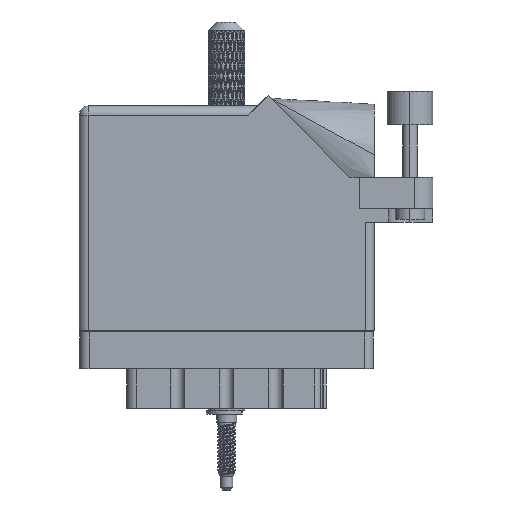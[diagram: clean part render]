
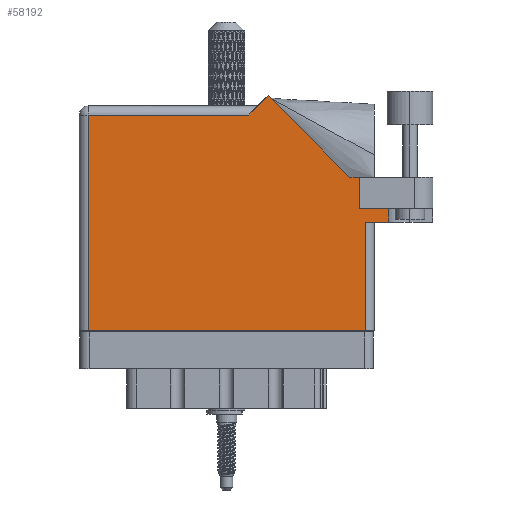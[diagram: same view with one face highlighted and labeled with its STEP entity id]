
A CAD part, front view. The second image highlights one B-rep face of the part: STEP entity #58192.
In plain terms, the highlighted face is planar.
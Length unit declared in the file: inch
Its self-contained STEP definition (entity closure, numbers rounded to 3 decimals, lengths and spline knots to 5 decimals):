
#96 = VECTOR ( 'NONE', #58342, 39.37008 ) ;
#247 = EDGE_CURVE ( 'NONE', #43957, #99186, #44743, .T. ) ;
#1475 = VERTEX_POINT ( 'NONE', #89538 ) ;
#3859 = LINE ( 'NONE', #57505, #86790 ) ;
#4360 = VECTOR ( 'NONE', #66414, 39.37008 ) ;
#4666 = CARTESIAN_POINT ( 'NONE',  ( 1.948, 0.737, 0. ) ) ;
#5744 = VERTEX_POINT ( 'NONE', #47094 ) ;
#8907 = CARTESIAN_POINT ( 'NONE',  ( 0.062, 0., 0. ) ) ;
#10261 = CARTESIAN_POINT ( 'NONE',  ( 2.41, 1.044, 0. ) ) ;
#13015 = DIRECTION ( 'NONE',  ( 0., 1., 0. ) ) ;
#15179 = CARTESIAN_POINT ( 'NONE',  ( 1.948, 0.737, 0. ) ) ;
#17141 = CARTESIAN_POINT ( 'NONE',  ( 1.155, 1.468, 0. ) ) ;
#17288 = VECTOR ( 'NONE', #83470, 39.37008 ) ;
#17927 = ORIENTED_EDGE ( 'NONE', *, *, #98427, .F. ) ;
#19640 = LINE ( 'NONE', #77623, #62447 ) ;
#21634 = ORIENTED_EDGE ( 'NONE', *, *, #247, .T. ) ;
#21904 = CARTESIAN_POINT ( 'NONE',  ( 0., 0., 0. ) ) ;
#21919 = VECTOR ( 'NONE', #69348, 39.37008 ) ;
#23807 = CARTESIAN_POINT ( 'NONE',  ( 1.28771, 1.60071, 0. ) ) ;
#26473 = CARTESIAN_POINT ( 'NONE',  ( 1.91, 0.831, 0. ) ) ;
#26623 = AXIS2_PLACEMENT_3D ( 'NONE', #48962, #105425, #56221 ) ;
#26885 = EDGE_CURVE ( 'NONE', #1475, #105498, #107430, .T. ) ;
#27562 = DIRECTION ( 'NONE',  ( -0.707, -0.707, 0. ) ) ;
#28063 = LINE ( 'NONE', #89338, #53928 ) ;
#28598 = ORIENTED_EDGE ( 'NONE', *, *, #95129, .T. ) ;
#28886 = CARTESIAN_POINT ( 'NONE',  ( 1.84442, 1.044, 0. ) ) ;
#30635 = LINE ( 'NONE', #65746, #93976 ) ;
#32898 = ORIENTED_EDGE ( 'NONE', *, *, #69110, .F. ) ;
#33162 = DIRECTION ( 'NONE',  ( 0., -1., 0. ) ) ;
#34593 = VERTEX_POINT ( 'NONE', #17141 ) ;
#36619 = CARTESIAN_POINT ( 'NONE',  ( 1.217, 1.53, 0. ) ) ;
#37528 = DIRECTION ( 'NONE',  ( 1., 0., 0. ) ) ;
#42921 = VECTOR ( 'NONE', #37528, 39.37008 ) ;
#43957 = VERTEX_POINT ( 'NONE', #69590 ) ;
#44743 = LINE ( 'NONE', #4666, #57774 ) ;
#45487 = LINE ( 'NONE', #21904, #42921 ) ;
#45895 = EDGE_CURVE ( 'NONE', #105498, #94994, #79507, .T. ) ;
#47094 = CARTESIAN_POINT ( 'NONE',  ( 0.062, 1.468, 0. ) ) ;
#47248 = FACE_OUTER_BOUND ( 'NONE', #101549, .T. ) ;
#48962 = CARTESIAN_POINT ( 'NONE',  ( 0., 1.53, 0. ) ) ;
#50933 = ORIENTED_EDGE ( 'NONE', *, *, #80934, .T. ) ;
#52217 = VERTEX_POINT ( 'NONE', #100976 ) ;
#53928 = VECTOR ( 'NONE', #88274, 39.37008 ) ;
#54864 = LINE ( 'NONE', #88343, #96 ) ;
#55256 = EDGE_CURVE ( 'NONE', #94994, #34593, #92895, .T. ) ;
#55393 = VERTEX_POINT ( 'NONE', #55421 ) ;
#55421 = CARTESIAN_POINT ( 'NONE',  ( 2.1115, 0.737, 0. ) ) ;
#56221 = DIRECTION ( 'NONE',  ( -1., 0., 0. ) ) ;
#57505 = CARTESIAN_POINT ( 'NONE',  ( 1.91, 0.831, 0. ) ) ;
#57774 = VECTOR ( 'NONE', #13015, 39.37008 ) ;
#58192 = ADVANCED_FACE ( 'NONE', ( #47248 ), #71475, .F. ) ;
#58342 = DIRECTION ( 'NONE',  ( 0., 1., 0. ) ) ;
#58554 = ORIENTED_EDGE ( 'NONE', *, *, #105888, .T. ) ;
#62447 = VECTOR ( 'NONE', #70772, 39.37008 ) ;
#65503 = ORIENTED_EDGE ( 'NONE', *, *, #86765, .T. ) ;
#65746 = CARTESIAN_POINT ( 'NONE',  ( 0.062, 0., 0. ) ) ;
#66414 = DIRECTION ( 'NONE',  ( -0.707, 0.707, 0. ) ) ;
#69110 = EDGE_CURVE ( 'NONE', #52217, #55393, #28063, .T. ) ;
#69348 = DIRECTION ( 'NONE',  ( -1., 0., 0. ) ) ;
#69590 = CARTESIAN_POINT ( 'NONE',  ( 1.948, 0., 0. ) ) ;
#70772 = DIRECTION ( 'NONE',  ( -1., 0., 0. ) ) ;
#70841 = ORIENTED_EDGE ( 'NONE', *, *, #26885, .T. ) ;
#71445 = VERTEX_POINT ( 'NONE', #8907 ) ;
#71475 = PLANE ( 'NONE',  #26623 ) ;
#77623 = CARTESIAN_POINT ( 'NONE',  ( 0., 1.468, 0. ) ) ;
#79507 = LINE ( 'NONE', #100362, #4360 ) ;
#80934 = EDGE_CURVE ( 'NONE', #71445, #43957, #45487, .T. ) ;
#82495 = VECTOR ( 'NONE', #27562, 39.37008 ) ;
#83470 = DIRECTION ( 'NONE',  ( 1., 0., 0. ) ) ;
#86765 = EDGE_CURVE ( 'NONE', #5744, #71445, #30635, .T. ) ;
#86790 = VECTOR ( 'NONE', #90725, 39.37008 ) ;
#88274 = DIRECTION ( 'NONE',  ( 0., -1., 0. ) ) ;
#88343 = CARTESIAN_POINT ( 'NONE',  ( 1.91, 0.831, 0. ) ) ;
#89338 = CARTESIAN_POINT ( 'NONE',  ( 2.1115, 1.16177, 0. ) ) ;
#89538 = CARTESIAN_POINT ( 'NONE',  ( 1.91, 1.044, 0. ) ) ;
#89957 = VERTEX_POINT ( 'NONE', #26473 ) ;
#90725 = DIRECTION ( 'NONE',  ( 1., 0., 0. ) ) ;
#90883 = ORIENTED_EDGE ( 'NONE', *, *, #45895, .T. ) ;
#92517 = CARTESIAN_POINT ( 'NONE',  ( 2.01, 0.737, 0. ) ) ;
#92891 = ORIENTED_EDGE ( 'NONE', *, *, #100277, .T. ) ;
#92895 = LINE ( 'NONE', #36619, #82495 ) ;
#93976 = VECTOR ( 'NONE', #33162, 39.37008 ) ;
#94982 = LINE ( 'NONE', #92517, #17288 ) ;
#94994 = VERTEX_POINT ( 'NONE', #23807 ) ;
#95129 = EDGE_CURVE ( 'NONE', #99186, #55393, #94982, .T. ) ;
#98427 = EDGE_CURVE ( 'NONE', #89957, #52217, #3859, .T. ) ;
#99186 = VERTEX_POINT ( 'NONE', #15179 ) ;
#100277 = EDGE_CURVE ( 'NONE', #89957, #1475, #54864, .T. ) ;
#100362 = CARTESIAN_POINT ( 'NONE',  ( 1.84442, 1.044, 0. ) ) ;
#100976 = CARTESIAN_POINT ( 'NONE',  ( 2.1115, 0.831, 0. ) ) ;
#101549 = EDGE_LOOP ( 'NONE', ( #50933, #21634, #28598, #32898, #17927, #92891, #70841, #90883, #104343, #58554, #65503 ) ) ;
#104343 = ORIENTED_EDGE ( 'NONE', *, *, #55256, .T. ) ;
#105425 = DIRECTION ( 'NONE',  ( 0., 0., -1. ) ) ;
#105498 = VERTEX_POINT ( 'NONE', #28886 ) ;
#105888 = EDGE_CURVE ( 'NONE', #34593, #5744, #19640, .T. ) ;
#107430 = LINE ( 'NONE', #10261, #21919 ) ;
